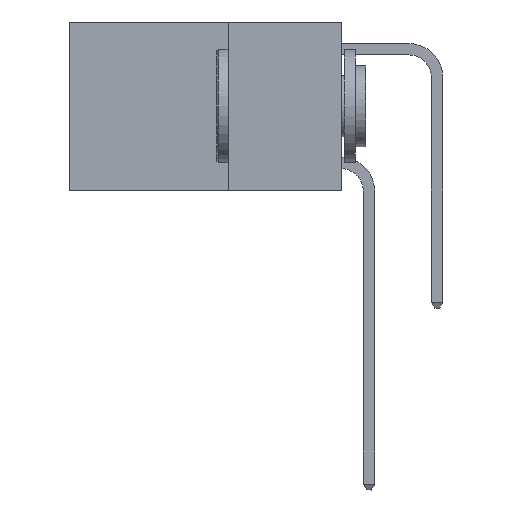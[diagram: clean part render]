
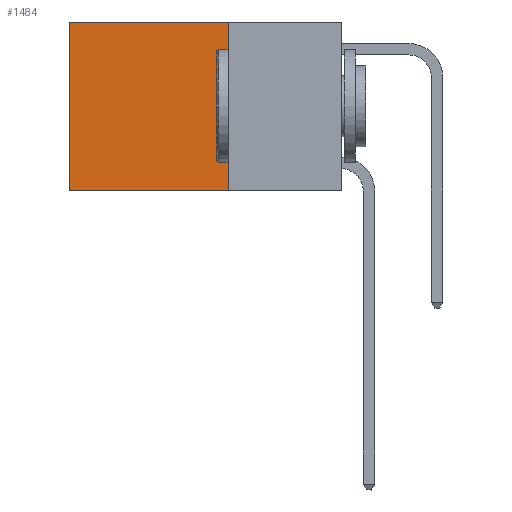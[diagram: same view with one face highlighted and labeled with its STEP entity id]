
A CAD part, left-side view. The second image highlights one B-rep face of the part: STEP entity #1484.
In plain terms, the highlighted planar face has unit normal (-1, 0, 0).
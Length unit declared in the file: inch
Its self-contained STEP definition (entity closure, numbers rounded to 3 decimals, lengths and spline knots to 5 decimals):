
#176 = CARTESIAN_POINT ( 'NONE',  ( 0.2625, 0.25, 0. ) ) ;
#770 = VECTOR ( 'NONE', #1492, 39.37008 ) ;
#787 = EDGE_CURVE ( 'NONE', #4833, #8069, #9659, .T. ) ;
#1143 = EDGE_CURVE ( 'NONE', #8069, #6226, #5274, .T. ) ;
#1484 = ADVANCED_FACE ( 'NONE', ( #13224 ), #2811, .F. ) ;
#1492 = DIRECTION ( 'NONE',  ( 0., 1., 0. ) ) ;
#2726 = DIRECTION ( 'NONE',  ( 0., 0., -1. ) ) ;
#2742 = DIRECTION ( 'NONE',  ( 1., 0., 0. ) ) ;
#2811 = PLANE ( 'NONE',  #4140 ) ;
#3063 = CARTESIAN_POINT ( 'NONE',  ( 0.2625, 0.25, 0. ) ) ;
#3289 = CARTESIAN_POINT ( 'NONE',  ( 0.2625, 0.6, 0. ) ) ;
#3633 = DIRECTION ( 'NONE',  ( 0., 0., -1. ) ) ;
#4140 = AXIS2_PLACEMENT_3D ( 'NONE', #3063, #2742, #2726 ) ;
#4233 = CARTESIAN_POINT ( 'NONE',  ( 0.2625, 0.25, -0.37 ) ) ;
#4248 = LINE ( 'NONE', #176, #770 ) ;
#4833 = VERTEX_POINT ( 'NONE', #12345 ) ;
#5274 = LINE ( 'NONE', #4233, #7887 ) ;
#6029 = ORIENTED_EDGE ( 'NONE', *, *, #8014, .T. ) ;
#6044 = ORIENTED_EDGE ( 'NONE', *, *, #1143, .F. ) ;
#6098 = CARTESIAN_POINT ( 'NONE',  ( 0.2625, 0.6, -0.37 ) ) ;
#6198 = EDGE_LOOP ( 'NONE', ( #6029, #6044, #7885, #7840 ) ) ;
#6226 = VERTEX_POINT ( 'NONE', #6098 ) ;
#7840 = ORIENTED_EDGE ( 'NONE', *, *, #10786, .T. ) ;
#7885 = ORIENTED_EDGE ( 'NONE', *, *, #787, .F. ) ;
#7887 = VECTOR ( 'NONE', #8316, 39.37008 ) ;
#7988 = VECTOR ( 'NONE', #10941, 39.37008 ) ;
#8014 = EDGE_CURVE ( 'NONE', #12461, #6226, #11302, .T. ) ;
#8069 = VERTEX_POINT ( 'NONE', #9854 ) ;
#8316 = DIRECTION ( 'NONE',  ( 0., 1., 0. ) ) ;
#9253 = CARTESIAN_POINT ( 'NONE',  ( 0.2625, 0.6, 0. ) ) ;
#9659 = LINE ( 'NONE', #12645, #15429 ) ;
#9854 = CARTESIAN_POINT ( 'NONE',  ( 0.2625, 0.25, -0.37 ) ) ;
#10786 = EDGE_CURVE ( 'NONE', #4833, #12461, #4248, .T. ) ;
#10941 = DIRECTION ( 'NONE',  ( 0., 0., -1. ) ) ;
#11302 = LINE ( 'NONE', #3289, #7988 ) ;
#12345 = CARTESIAN_POINT ( 'NONE',  ( 0.2625, 0.25, 0. ) ) ;
#12461 = VERTEX_POINT ( 'NONE', #9253 ) ;
#12645 = CARTESIAN_POINT ( 'NONE',  ( 0.2625, 0.25, 0. ) ) ;
#13224 = FACE_OUTER_BOUND ( 'NONE', #6198, .T. ) ;
#15429 = VECTOR ( 'NONE', #3633, 39.37008 ) ;
